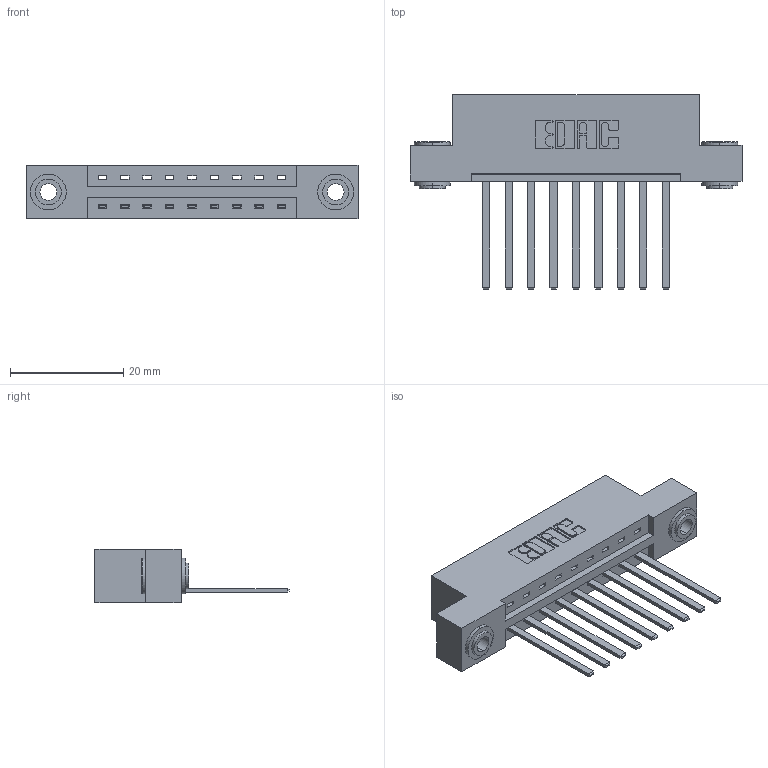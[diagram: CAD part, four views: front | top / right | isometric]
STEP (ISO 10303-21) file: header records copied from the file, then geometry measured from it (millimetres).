
FILE_DESCRIPTION (( 'STEP AP203' ), '1' );
FILE_NAME ('337-009-544-103.STEP', '2018-08-03T22:59:07', ( '' ), ( '' ), 'SwSTEP 2.0', 'SolidWorks 2016', '' );
FILE_SCHEMA (( 'CONFIG_CONTROL_DESIGN' ));
Length unit declared in the file: inch
Products named in the file (4): 337 Part_Flush Mounting Lugs - 0.156 Dia-TH; 345-292-001_345-293-144; 345-250-002_345-250-002-102; 337-009-544-103
Assembly tree (12 placements, depth 2):
  337-009-544-103
    337 Part_Flush Mounting Lugs - 0.156 Dia-TH
    345-292-001_345-293-144  x9
    345-250-002_345-250-002-102  x2
Bounding box: 58.67 x 34.3 x 9.4 mm (x, y, z)
Volume: 5808.8 mm3; surface area: 6395 mm2
Topology: 12 solids, 12 shells, 656 faces, 1917 edges, 1262 vertices
Faces by surface type: plane 458, cylinder 190, cone 8
Entity records: 11424 total; most frequent: CARTESIAN_POINT 1964, ORIENTED_EDGE 1902, DIRECTION 1751, EDGE_CURVE 951, VECTOR 803, LINE 803, VERTEX_POINT 630, AXIS2_PLACEMENT_3D 474
